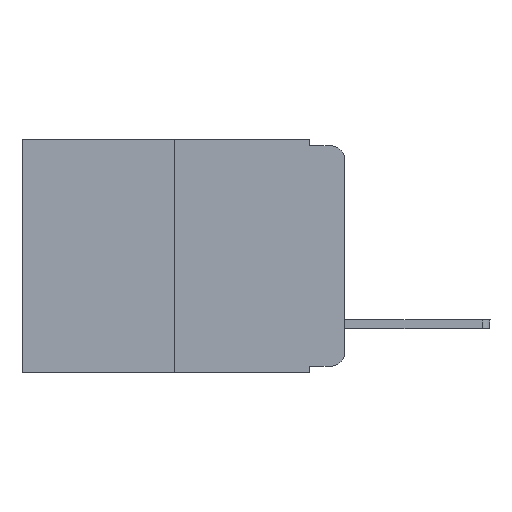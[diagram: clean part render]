
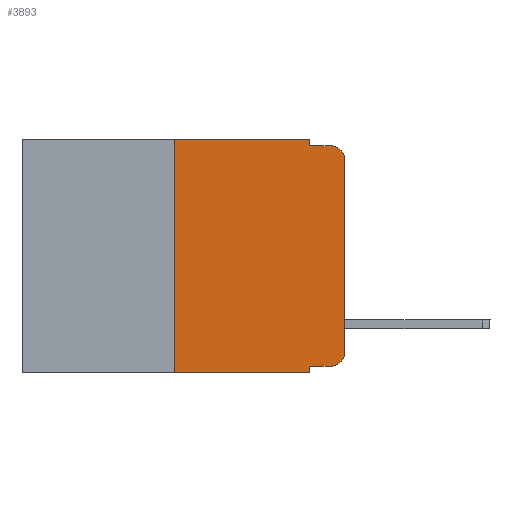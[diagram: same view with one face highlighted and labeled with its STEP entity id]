
A CAD part, left-side view. The second image highlights one B-rep face of the part: STEP entity #3893.
In plain terms, the highlighted planar face has unit normal (-1, 0, 0).
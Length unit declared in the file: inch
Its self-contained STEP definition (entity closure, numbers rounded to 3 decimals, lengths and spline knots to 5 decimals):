
#143 = VECTOR ( 'NONE', #9685, 39.37008 ) ;
#532 = VERTEX_POINT ( 'NONE', #5666 ) ;
#604 = CARTESIAN_POINT ( 'NONE',  ( 0., 0.02, -0.03 ) ) ;
#656 = LINE ( 'NONE', #8386, #143 ) ;
#894 = PLANE ( 'NONE',  #14162 ) ;
#972 = CARTESIAN_POINT ( 'NONE',  ( 0., 0.473, 0. ) ) ;
#1421 = CIRCLE ( 'NONE', #14225, 0.02 ) ;
#1452 = DIRECTION ( 'NONE',  ( 0., 0., -1. ) ) ;
#1602 = CARTESIAN_POINT ( 'NONE',  ( 0., 0., -0.03 ) ) ;
#1676 = EDGE_CURVE ( 'NONE', #6531, #10572, #656, .T. ) ;
#1754 = CARTESIAN_POINT ( 'NONE',  ( 0., 0.02, -0.313 ) ) ;
#2163 = VECTOR ( 'NONE', #13818, 39.37008 ) ;
#2558 = VECTOR ( 'NONE', #14138, 39.37008 ) ;
#2913 = CARTESIAN_POINT ( 'NONE',  ( 0., 0.473, -0.343 ) ) ;
#3070 = VECTOR ( 'NONE', #1452, 39.37008 ) ;
#3358 = VERTEX_POINT ( 'NONE', #1602 ) ;
#3793 = ORIENTED_EDGE ( 'NONE', *, *, #13648, .T. ) ;
#3893 = ADVANCED_FACE ( 'NONE', ( #10891 ), #894, .F. ) ;
#4175 = DIRECTION ( 'NONE',  ( -1., 0., 0. ) ) ;
#4196 = CARTESIAN_POINT ( 'NONE',  ( 0., 0.25, 0. ) ) ;
#4239 = VECTOR ( 'NONE', #8340, 39.37008 ) ;
#4656 = CARTESIAN_POINT ( 'NONE',  ( 0., 0.051, -0.01 ) ) ;
#5135 = CARTESIAN_POINT ( 'NONE',  ( 0., 0.051, -0.333 ) ) ;
#5287 = CARTESIAN_POINT ( 'NONE',  ( 0., 0.051, 0. ) ) ;
#5552 = LINE ( 'NONE', #13231, #6135 ) ;
#5666 = CARTESIAN_POINT ( 'NONE',  ( 0., 0.25, -0.343 ) ) ;
#6135 = VECTOR ( 'NONE', #9771, 39.37008 ) ;
#6136 = DIRECTION ( 'NONE',  ( -1., 0., 0. ) ) ;
#6321 = EDGE_CURVE ( 'NONE', #532, #6531, #11154, .T. ) ;
#6437 = VERTEX_POINT ( 'NONE', #11586 ) ;
#6531 = VERTEX_POINT ( 'NONE', #4196 ) ;
#6598 = ORIENTED_EDGE ( 'NONE', *, *, #13178, .F. ) ;
#7008 = VECTOR ( 'NONE', #13423, 39.37008 ) ;
#7118 = ORIENTED_EDGE ( 'NONE', *, *, #1676, .F. ) ;
#7215 = DIRECTION ( 'NONE',  ( 0., 0., -1. ) ) ;
#7289 = EDGE_CURVE ( 'NONE', #8957, #6437, #13298, .T. ) ;
#7384 = DIRECTION ( 'NONE',  ( 0., 0., -1. ) ) ;
#7420 = VERTEX_POINT ( 'NONE', #9826 ) ;
#7465 = LINE ( 'NONE', #5135, #4239 ) ;
#7643 = EDGE_LOOP ( 'NONE', ( #10825, #9033, #9394, #12705, #7118, #7989, #8610, #6598, #3793, #12528 ) ) ;
#7816 = VERTEX_POINT ( 'NONE', #9587 ) ;
#7896 = VERTEX_POINT ( 'NONE', #12974 ) ;
#7989 = ORIENTED_EDGE ( 'NONE', *, *, #6321, .F. ) ;
#8041 = CARTESIAN_POINT ( 'NONE',  ( 0., 0.051, 0. ) ) ;
#8340 = DIRECTION ( 'NONE',  ( 0., -1., 0. ) ) ;
#8386 = CARTESIAN_POINT ( 'NONE',  ( 0., 0.473, 0. ) ) ;
#8530 = VERTEX_POINT ( 'NONE', #4656 ) ;
#8545 = DIRECTION ( 'NONE',  ( 1., 0., 0. ) ) ;
#8610 = ORIENTED_EDGE ( 'NONE', *, *, #9758, .T. ) ;
#8944 = CARTESIAN_POINT ( 'NONE',  ( 0., 0.25, 0. ) ) ;
#8957 = VERTEX_POINT ( 'NONE', #13480 ) ;
#9033 = ORIENTED_EDGE ( 'NONE', *, *, #12229, .T. ) ;
#9394 = ORIENTED_EDGE ( 'NONE', *, *, #14241, .F. ) ;
#9563 = DIRECTION ( 'NONE',  ( 0., 0., 1. ) ) ;
#9587 = CARTESIAN_POINT ( 'NONE',  ( 0., 0.02, -0.01 ) ) ;
#9685 = DIRECTION ( 'NONE',  ( 0., -1., 0. ) ) ;
#9758 = EDGE_CURVE ( 'NONE', #532, #7420, #12123, .T. ) ;
#9771 = DIRECTION ( 'NONE',  ( 0., -1., 0. ) ) ;
#9826 = CARTESIAN_POINT ( 'NONE',  ( 0., 0.051, -0.343 ) ) ;
#10225 = LINE ( 'NONE', #8041, #2163 ) ;
#10336 = LINE ( 'NONE', #11443, #3070 ) ;
#10572 = VERTEX_POINT ( 'NONE', #5287 ) ;
#10746 = LINE ( 'NONE', #12809, #11210 ) ;
#10825 = ORIENTED_EDGE ( 'NONE', *, *, #10975, .T. ) ;
#10891 = FACE_OUTER_BOUND ( 'NONE', #7643, .T. ) ;
#10975 = EDGE_CURVE ( 'NONE', #6437, #3358, #10746, .T. ) ;
#11154 = LINE ( 'NONE', #8944, #7008 ) ;
#11210 = VECTOR ( 'NONE', #9563, 39.37008 ) ;
#11443 = CARTESIAN_POINT ( 'NONE',  ( 0., 0.051, 0. ) ) ;
#11586 = CARTESIAN_POINT ( 'NONE',  ( 0., 0., -0.313 ) ) ;
#12123 = LINE ( 'NONE', #2913, #2558 ) ;
#12215 = AXIS2_PLACEMENT_3D ( 'NONE', #1754, #6136, #7215 ) ;
#12229 = EDGE_CURVE ( 'NONE', #3358, #7816, #1421, .T. ) ;
#12528 = ORIENTED_EDGE ( 'NONE', *, *, #7289, .T. ) ;
#12705 = ORIENTED_EDGE ( 'NONE', *, *, #13968, .F. ) ;
#12809 = CARTESIAN_POINT ( 'NONE',  ( 0., 0., 0. ) ) ;
#12974 = CARTESIAN_POINT ( 'NONE',  ( 0., 0.051, -0.333 ) ) ;
#13178 = EDGE_CURVE ( 'NONE', #7896, #7420, #10336, .T. ) ;
#13231 = CARTESIAN_POINT ( 'NONE',  ( 0., 0.051, -0.01 ) ) ;
#13298 = CIRCLE ( 'NONE', #12215, 0.02 ) ;
#13319 = DIRECTION ( 'NONE',  ( 0., 0., -1. ) ) ;
#13423 = DIRECTION ( 'NONE',  ( 0., 0., 1. ) ) ;
#13480 = CARTESIAN_POINT ( 'NONE',  ( 0., 0.02, -0.333 ) ) ;
#13648 = EDGE_CURVE ( 'NONE', #7896, #8957, #7465, .T. ) ;
#13818 = DIRECTION ( 'NONE',  ( 0., 0., -1. ) ) ;
#13968 = EDGE_CURVE ( 'NONE', #10572, #8530, #10225, .T. ) ;
#14138 = DIRECTION ( 'NONE',  ( 0., -1., 0. ) ) ;
#14162 = AXIS2_PLACEMENT_3D ( 'NONE', #972, #8545, #13319 ) ;
#14225 = AXIS2_PLACEMENT_3D ( 'NONE', #604, #4175, #7384 ) ;
#14241 = EDGE_CURVE ( 'NONE', #8530, #7816, #5552, .T. ) ;
